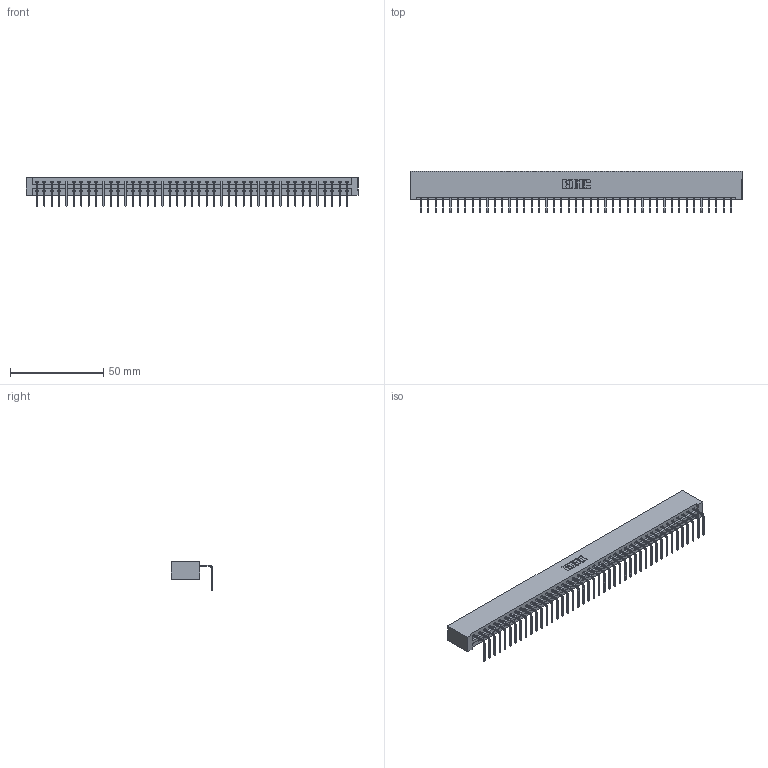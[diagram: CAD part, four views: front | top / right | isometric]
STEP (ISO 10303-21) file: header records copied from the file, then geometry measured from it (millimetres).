
FILE_DESCRIPTION (( 'STEP AP203' ), '1' );
FILE_NAME ('387-043-558-101.STEP', '2018-09-20T01:15:44', ( '' ), ( '' ), 'SwSTEP 2.0', 'SolidWorks 2016', '' );
FILE_SCHEMA (( 'CONFIG_CONTROL_DESIGN' ));
Length unit declared in the file: inch
Products named in the file (3): 337 Part_No Mounting Lugs; 345-292-001_558 Tail - 2; 387-043-558-101
Assembly tree (44 placements, depth 2):
  387-043-558-101
    337 Part_No Mounting Lugs
    345-292-001_558 Tail - 2  x43
Bounding box: 178.26 x 22.17 x 15.37 mm (x, y, z)
Volume: 19421.3 mm3; surface area: 20936.2 mm2
Topology: 44 solids, 44 shells, 2858 faces, 8629 edges, 5694 vertices
Faces by surface type: plane 2130, cylinder 728
Entity records: 31641 total; most frequent: CARTESIAN_POINT 5519, ORIENTED_EDGE 5498, DIRECTION 4635, EDGE_CURVE 2749, VECTOR 2629, LINE 2629, VERTEX_POINT 1830, AXIS2_PLACEMENT_3D 1003
